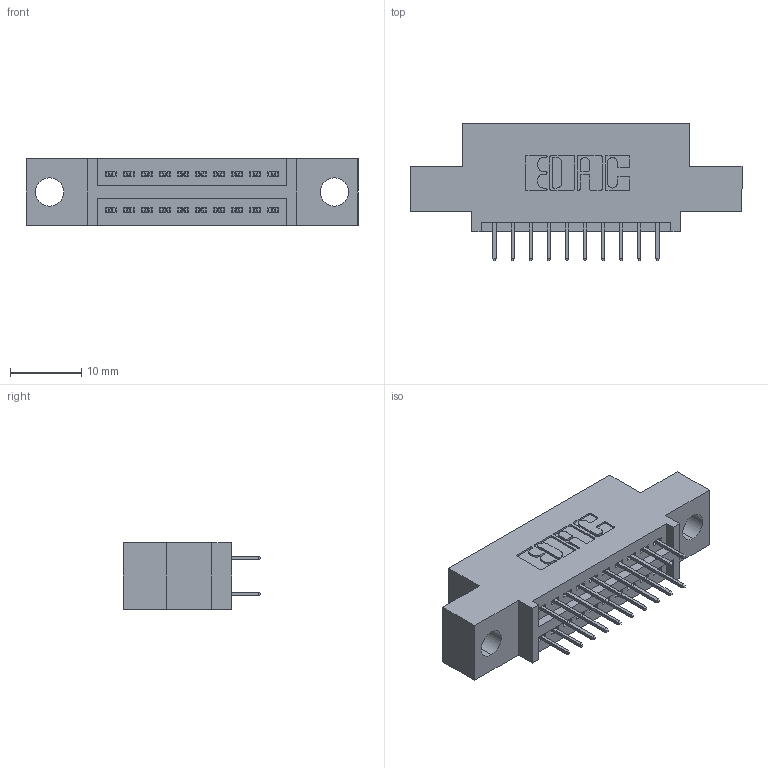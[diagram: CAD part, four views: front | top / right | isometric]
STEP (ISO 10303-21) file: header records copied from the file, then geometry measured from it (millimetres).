
FILE_DESCRIPTION (( 'STEP AP203' ), '1' );
FILE_NAME ('345-020-524-504.STEP', '2021-05-19T21:49:15', ( '' ), ( '' ), 'SwSTEP 2.0', 'SolidWorks 2020', '' );
FILE_SCHEMA (( 'CONFIG_CONTROL_DESIGN' ));
Length unit declared in the file: inch
Products named in the file (3): 345 Part_0.110 Offset - 0.156 Dia-TI; 345-020-524-504; 345-292-001_345-293-124
Assembly tree (21 placements, depth 2):
  345-020-524-504
    345 Part_0.110 Offset - 0.156 Dia-TI
    345-292-001_345-293-124  x20
Bounding box: 46.61 x 19.35 x 9.4 mm (x, y, z)
Volume: 4021 mm3; surface area: 5188.5 mm2
Topology: 21 solids, 21 shells, 1224 faces, 3449 edges, 2218 vertices
Faces by surface type: plane 878, cylinder 346
Entity records: 12779 total; most frequent: CARTESIAN_POINT 2178, ORIENTED_EDGE 2110, DIRECTION 1959, EDGE_CURVE 1055, VECTOR 887, LINE 887, VERTEX_POINT 698, AXIS2_PLACEMENT_3D 536
